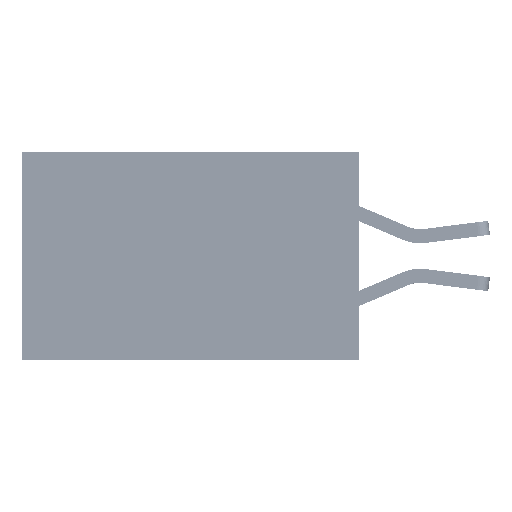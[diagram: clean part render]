
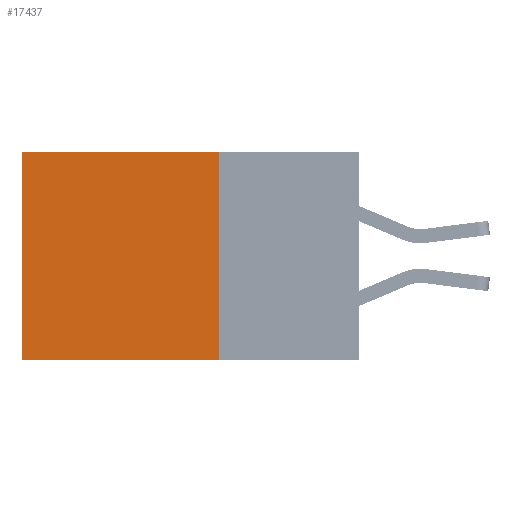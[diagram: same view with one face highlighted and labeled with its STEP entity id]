
A CAD part, left-side view. The second image highlights one B-rep face of the part: STEP entity #17437.
In plain terms, the highlighted planar face has unit normal (-1, 0, 0).
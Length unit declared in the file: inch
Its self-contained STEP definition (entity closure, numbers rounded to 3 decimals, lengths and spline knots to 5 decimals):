
#63 = CARTESIAN_POINT ( 'NONE',  ( 0.2875, 0.25, 0. ) ) ;
#363 = LINE ( 'NONE', #4225, #31528 ) ;
#377 = CARTESIAN_POINT ( 'NONE',  ( 0.2875, 0.25, -0.37 ) ) ;
#1993 = EDGE_CURVE ( 'NONE', #5777, #5539, #33909, .T. ) ;
#2176 = VECTOR ( 'NONE', #24661, 39.37008 ) ;
#3782 = ORIENTED_EDGE ( 'NONE', *, *, #1993, .F. ) ;
#3983 = CARTESIAN_POINT ( 'NONE',  ( 0.2875, 0.6, 0. ) ) ;
#4225 = CARTESIAN_POINT ( 'NONE',  ( 0.2875, 0.25, 0. ) ) ;
#4914 = ORIENTED_EDGE ( 'NONE', *, *, #6310, .T. ) ;
#5048 = EDGE_CURVE ( 'NONE', #26705, #5777, #23282, .T. ) ;
#5539 = VERTEX_POINT ( 'NONE', #10723 ) ;
#5777 = VERTEX_POINT ( 'NONE', #377 ) ;
#6310 = EDGE_CURVE ( 'NONE', #26705, #14042, #363, .T. ) ;
#9813 = VECTOR ( 'NONE', #17682, 39.37008 ) ;
#10202 = DIRECTION ( 'NONE',  ( 0., 1., 0. ) ) ;
#10435 = PLANE ( 'NONE',  #12899 ) ;
#10723 = CARTESIAN_POINT ( 'NONE',  ( 0.2875, 0.6, -0.37 ) ) ;
#11116 = ORIENTED_EDGE ( 'NONE', *, *, #5048, .F. ) ;
#12324 = CARTESIAN_POINT ( 'NONE',  ( 0.2875, 0.6, 0. ) ) ;
#12899 = AXIS2_PLACEMENT_3D ( 'NONE', #13421, #34178, #37125 ) ;
#13421 = CARTESIAN_POINT ( 'NONE',  ( 0.2875, 0.25, 0. ) ) ;
#14042 = VERTEX_POINT ( 'NONE', #12324 ) ;
#14074 = CARTESIAN_POINT ( 'NONE',  ( 0.2875, 0.25, 0. ) ) ;
#15574 = LINE ( 'NONE', #3983, #2176 ) ;
#15793 = EDGE_LOOP ( 'NONE', ( #24474, #3782, #11116, #4914 ) ) ;
#16255 = VECTOR ( 'NONE', #21307, 39.37008 ) ;
#17437 = ADVANCED_FACE ( 'NONE', ( #21046 ), #10435, .F. ) ;
#17682 = DIRECTION ( 'NONE',  ( 0., 0., -1. ) ) ;
#21046 = FACE_OUTER_BOUND ( 'NONE', #15793, .T. ) ;
#21307 = DIRECTION ( 'NONE',  ( 0., 1., 0. ) ) ;
#23282 = LINE ( 'NONE', #63, #9813 ) ;
#24474 = ORIENTED_EDGE ( 'NONE', *, *, #27361, .T. ) ;
#24661 = DIRECTION ( 'NONE',  ( 0., 0., -1. ) ) ;
#26705 = VERTEX_POINT ( 'NONE', #14074 ) ;
#27361 = EDGE_CURVE ( 'NONE', #14042, #5539, #15574, .T. ) ;
#29946 = CARTESIAN_POINT ( 'NONE',  ( 0.2875, 0.25, -0.37 ) ) ;
#31528 = VECTOR ( 'NONE', #10202, 39.37008 ) ;
#33909 = LINE ( 'NONE', #29946, #16255 ) ;
#34178 = DIRECTION ( 'NONE',  ( 1., 0., 0. ) ) ;
#37125 = DIRECTION ( 'NONE',  ( 0., 0., -1. ) ) ;
